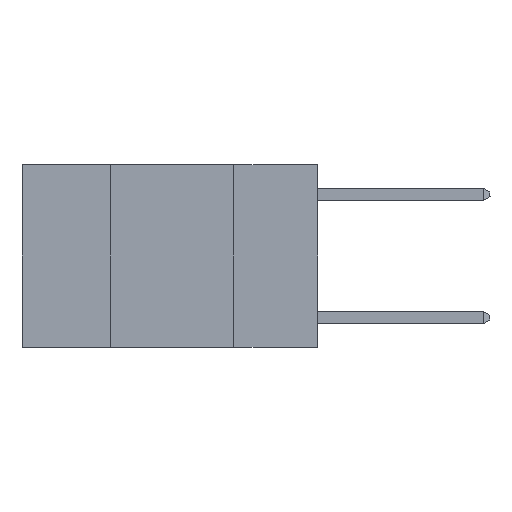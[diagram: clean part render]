
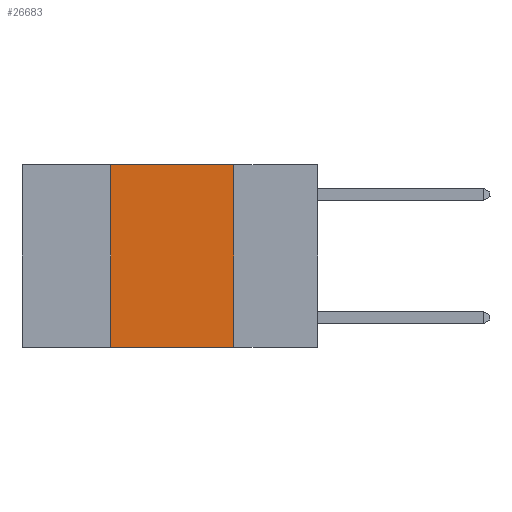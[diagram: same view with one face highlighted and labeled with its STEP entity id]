
A CAD part, left-side view. The second image highlights one B-rep face of the part: STEP entity #26683.
In plain terms, the highlighted planar face has unit normal (-1, 0, 0).
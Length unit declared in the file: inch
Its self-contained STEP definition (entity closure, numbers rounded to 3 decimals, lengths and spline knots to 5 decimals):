
#468 = CARTESIAN_POINT ( 'NONE',  ( 0., 0.42, -0.37 ) ) ;
#1132 = EDGE_CURVE ( 'NONE', #1519, #9836, #8635, .T. ) ;
#1519 = VERTEX_POINT ( 'NONE', #2989 ) ;
#2989 = CARTESIAN_POINT ( 'NONE',  ( 0., 0.17, 0. ) ) ;
#3167 = CARTESIAN_POINT ( 'NONE',  ( 0., 0.17, -0.37 ) ) ;
#5979 = CARTESIAN_POINT ( 'NONE',  ( 0., 0.17, 0. ) ) ;
#8180 = CARTESIAN_POINT ( 'NONE',  ( 0., 0.6, 0. ) ) ;
#8635 = LINE ( 'NONE', #5979, #26651 ) ;
#9836 = VERTEX_POINT ( 'NONE', #3167 ) ;
#9944 = EDGE_CURVE ( 'NONE', #18024, #23140, #14174, .T. ) ;
#10544 = DIRECTION ( 'NONE',  ( 0., -1., 0. ) ) ;
#10914 = PLANE ( 'NONE',  #20033 ) ;
#11015 = VECTOR ( 'NONE', #10544, 39.37008 ) ;
#11055 = LINE ( 'NONE', #18784, #29029 ) ;
#11168 = EDGE_CURVE ( 'NONE', #23140, #1519, #29724, .T. ) ;
#13327 = DIRECTION ( 'NONE',  ( 1., 0., 0. ) ) ;
#13488 = ORIENTED_EDGE ( 'NONE', *, *, #1132, .F. ) ;
#14174 = LINE ( 'NONE', #17664, #25896 ) ;
#14729 = ORIENTED_EDGE ( 'NONE', *, *, #11168, .F. ) ;
#14837 = ORIENTED_EDGE ( 'NONE', *, *, #9944, .F. ) ;
#15442 = DIRECTION ( 'NONE',  ( 0., 0., -1. ) ) ;
#16767 = ORIENTED_EDGE ( 'NONE', *, *, #26872, .T. ) ;
#17031 = FACE_OUTER_BOUND ( 'NONE', #19418, .T. ) ;
#17664 = CARTESIAN_POINT ( 'NONE',  ( 0., 0.42, 0. ) ) ;
#18024 = VERTEX_POINT ( 'NONE', #468 ) ;
#18784 = CARTESIAN_POINT ( 'NONE',  ( 0., 0.6, -0.37 ) ) ;
#19418 = EDGE_LOOP ( 'NONE', ( #13488, #14729, #14837, #16767 ) ) ;
#20023 = DIRECTION ( 'NONE',  ( 0., 0., 1. ) ) ;
#20033 = AXIS2_PLACEMENT_3D ( 'NONE', #27342, #13327, #29680 ) ;
#21159 = DIRECTION ( 'NONE',  ( 0., -1., 0. ) ) ;
#23140 = VERTEX_POINT ( 'NONE', #29668 ) ;
#25896 = VECTOR ( 'NONE', #20023, 39.37008 ) ;
#26651 = VECTOR ( 'NONE', #15442, 39.37008 ) ;
#26683 = ADVANCED_FACE ( 'NONE', ( #17031 ), #10914, .F. ) ;
#26872 = EDGE_CURVE ( 'NONE', #18024, #9836, #11055, .T. ) ;
#27342 = CARTESIAN_POINT ( 'NONE',  ( 0., 0.6, 0. ) ) ;
#29029 = VECTOR ( 'NONE', #21159, 39.37008 ) ;
#29668 = CARTESIAN_POINT ( 'NONE',  ( 0., 0.42, 0. ) ) ;
#29680 = DIRECTION ( 'NONE',  ( 0., 0., -1. ) ) ;
#29724 = LINE ( 'NONE', #8180, #11015 ) ;
